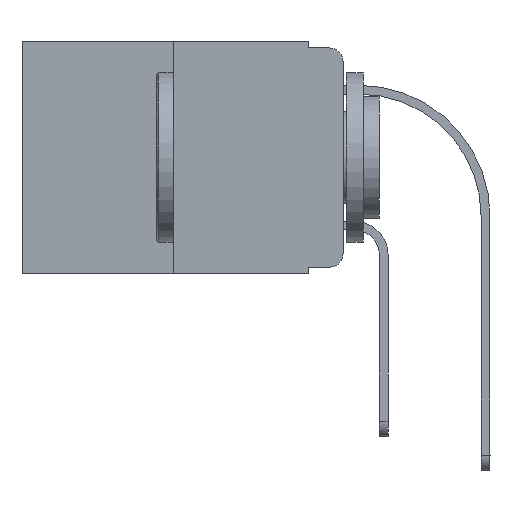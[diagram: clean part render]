
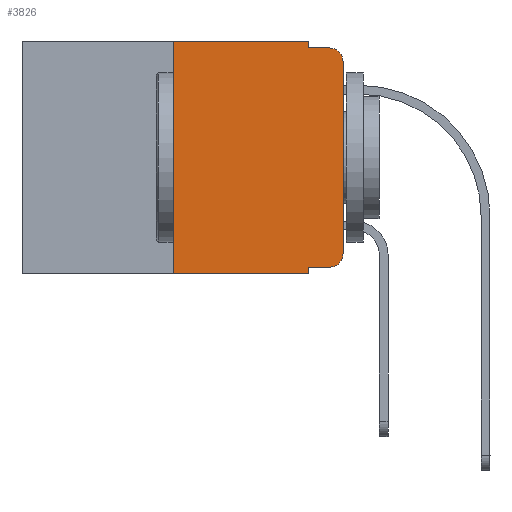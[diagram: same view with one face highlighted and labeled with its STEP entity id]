
A CAD part, left-side view. The second image highlights one B-rep face of the part: STEP entity #3826.
In plain terms, the highlighted planar face has unit normal (-1, 0, 0).
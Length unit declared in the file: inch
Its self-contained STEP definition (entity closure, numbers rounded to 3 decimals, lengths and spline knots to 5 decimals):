
#48 = AXIS2_PLACEMENT_3D ( 'NONE', #10967, #8844, #2830 ) ;
#68 = EDGE_CURVE ( 'NONE', #5214, #2494, #11411, .T. ) ;
#202 = VERTEX_POINT ( 'NONE', #5023 ) ;
#322 = VECTOR ( 'NONE', #10327, 39.37008 ) ;
#397 = VERTEX_POINT ( 'NONE', #2921 ) ;
#497 = VERTEX_POINT ( 'NONE', #11516 ) ;
#699 = VECTOR ( 'NONE', #8851, 39.37008 ) ;
#774 = ORIENTED_EDGE ( 'NONE', *, *, #12101, .T. ) ;
#1146 = ORIENTED_EDGE ( 'NONE', *, *, #4999, .F. ) ;
#1301 = EDGE_CURVE ( 'NONE', #497, #10928, #8979, .T. ) ;
#1470 = CARTESIAN_POINT ( 'NONE',  ( 0., 0., 0. ) ) ;
#1986 = CARTESIAN_POINT ( 'NONE',  ( 0., 0.473, 0. ) ) ;
#2088 = LINE ( 'NONE', #5087, #11263 ) ;
#2494 = VERTEX_POINT ( 'NONE', #7031 ) ;
#2599 = DIRECTION ( 'NONE',  ( 0., -1., 0. ) ) ;
#2830 = DIRECTION ( 'NONE',  ( 0., 0., -1. ) ) ;
#2921 = CARTESIAN_POINT ( 'NONE',  ( 0., 0.25, 0. ) ) ;
#3110 = CARTESIAN_POINT ( 'NONE',  ( 0., 0.473, 0. ) ) ;
#3291 = ORIENTED_EDGE ( 'NONE', *, *, #9948, .F. ) ;
#3474 = CARTESIAN_POINT ( 'NONE',  ( 0., 0.051, -0.01 ) ) ;
#3602 = DIRECTION ( 'NONE',  ( -1., 0., 0. ) ) ;
#3701 = EDGE_CURVE ( 'NONE', #2494, #3712, #6358, .T. ) ;
#3712 = VERTEX_POINT ( 'NONE', #6696 ) ;
#3826 = ADVANCED_FACE ( 'NONE', ( #11958 ), #7798, .F. ) ;
#3958 = CARTESIAN_POINT ( 'NONE',  ( 0., 0.051, -0.333 ) ) ;
#4040 = ORIENTED_EDGE ( 'NONE', *, *, #11387, .F. ) ;
#4674 = CARTESIAN_POINT ( 'NONE',  ( 0., 0.051, -0.333 ) ) ;
#4999 = EDGE_CURVE ( 'NONE', #6250, #10928, #8210, .T. ) ;
#5003 = DIRECTION ( 'NONE',  ( 1., 0., 0. ) ) ;
#5023 = CARTESIAN_POINT ( 'NONE',  ( 0., 0.051, -0.01 ) ) ;
#5087 = CARTESIAN_POINT ( 'NONE',  ( 0., 0.051, 0. ) ) ;
#5214 = VERTEX_POINT ( 'NONE', #8691 ) ;
#5701 = AXIS2_PLACEMENT_3D ( 'NONE', #6769, #3602, #12662 ) ;
#5715 = ORIENTED_EDGE ( 'NONE', *, *, #5916, .F. ) ;
#5842 = LINE ( 'NONE', #8875, #13005 ) ;
#5916 = EDGE_CURVE ( 'NONE', #497, #397, #5842, .T. ) ;
#6008 = CARTESIAN_POINT ( 'NONE',  ( 0., 0.473, -0.343 ) ) ;
#6100 = EDGE_CURVE ( 'NONE', #6250, #5214, #9535, .T. ) ;
#6250 = VERTEX_POINT ( 'NONE', #3958 ) ;
#6271 = VECTOR ( 'NONE', #2599, 39.37008 ) ;
#6358 = LINE ( 'NONE', #1470, #12797 ) ;
#6483 = ORIENTED_EDGE ( 'NONE', *, *, #6100, .T. ) ;
#6696 = CARTESIAN_POINT ( 'NONE',  ( 0., 0., -0.03 ) ) ;
#6769 = CARTESIAN_POINT ( 'NONE',  ( 0., 0.02, -0.313 ) ) ;
#7031 = CARTESIAN_POINT ( 'NONE',  ( 0., 0., -0.313 ) ) ;
#7068 = DIRECTION ( 'NONE',  ( 0., 0., -1. ) ) ;
#7263 = VECTOR ( 'NONE', #9880, 39.37008 ) ;
#7413 = ORIENTED_EDGE ( 'NONE', *, *, #1301, .T. ) ;
#7552 = VERTEX_POINT ( 'NONE', #11112 ) ;
#7753 = EDGE_CURVE ( 'NONE', #397, #13056, #8328, .T. ) ;
#7798 = PLANE ( 'NONE',  #7935 ) ;
#7872 = DIRECTION ( 'NONE',  ( 0., 0., 1. ) ) ;
#7877 = VECTOR ( 'NONE', #9458, 39.37008 ) ;
#7935 = AXIS2_PLACEMENT_3D ( 'NONE', #1986, #5003, #7068 ) ;
#8210 = LINE ( 'NONE', #12237, #322 ) ;
#8328 = LINE ( 'NONE', #3110, #7877 ) ;
#8578 = EDGE_LOOP ( 'NONE', ( #11274, #774, #3291, #4040, #8786, #5715, #7413, #1146, #6483, #12058 ) ) ;
#8691 = CARTESIAN_POINT ( 'NONE',  ( 0., 0.02, -0.333 ) ) ;
#8786 = ORIENTED_EDGE ( 'NONE', *, *, #7753, .F. ) ;
#8844 = DIRECTION ( 'NONE',  ( -1., 0., 0. ) ) ;
#8851 = DIRECTION ( 'NONE',  ( 0., -1., 0. ) ) ;
#8875 = CARTESIAN_POINT ( 'NONE',  ( 0., 0.25, 0. ) ) ;
#8886 = DIRECTION ( 'NONE',  ( 0., 0., -1. ) ) ;
#8979 = LINE ( 'NONE', #6008, #699 ) ;
#9458 = DIRECTION ( 'NONE',  ( 0., -1., 0. ) ) ;
#9535 = LINE ( 'NONE', #4674, #6271 ) ;
#9565 = LINE ( 'NONE', #3474, #7263 ) ;
#9880 = DIRECTION ( 'NONE',  ( 0., -1., 0. ) ) ;
#9948 = EDGE_CURVE ( 'NONE', #202, #7552, #9565, .T. ) ;
#10327 = DIRECTION ( 'NONE',  ( 0., 0., -1. ) ) ;
#10399 = DIRECTION ( 'NONE',  ( 0., 0., 1. ) ) ;
#10405 = CIRCLE ( 'NONE', #48, 0.02 ) ;
#10928 = VERTEX_POINT ( 'NONE', #11031 ) ;
#10967 = CARTESIAN_POINT ( 'NONE',  ( 0., 0.02, -0.03 ) ) ;
#11031 = CARTESIAN_POINT ( 'NONE',  ( 0., 0.051, -0.343 ) ) ;
#11112 = CARTESIAN_POINT ( 'NONE',  ( 0., 0.02, -0.01 ) ) ;
#11263 = VECTOR ( 'NONE', #8886, 39.37008 ) ;
#11274 = ORIENTED_EDGE ( 'NONE', *, *, #3701, .T. ) ;
#11387 = EDGE_CURVE ( 'NONE', #13056, #202, #2088, .T. ) ;
#11411 = CIRCLE ( 'NONE', #5701, 0.02 ) ;
#11516 = CARTESIAN_POINT ( 'NONE',  ( 0., 0.25, -0.343 ) ) ;
#11958 = FACE_OUTER_BOUND ( 'NONE', #8578, .T. ) ;
#12058 = ORIENTED_EDGE ( 'NONE', *, *, #68, .T. ) ;
#12092 = CARTESIAN_POINT ( 'NONE',  ( 0., 0.051, 0. ) ) ;
#12101 = EDGE_CURVE ( 'NONE', #3712, #7552, #10405, .T. ) ;
#12237 = CARTESIAN_POINT ( 'NONE',  ( 0., 0.051, 0. ) ) ;
#12662 = DIRECTION ( 'NONE',  ( 0., 0., -1. ) ) ;
#12797 = VECTOR ( 'NONE', #10399, 39.37008 ) ;
#13005 = VECTOR ( 'NONE', #7872, 39.37008 ) ;
#13056 = VERTEX_POINT ( 'NONE', #12092 ) ;
